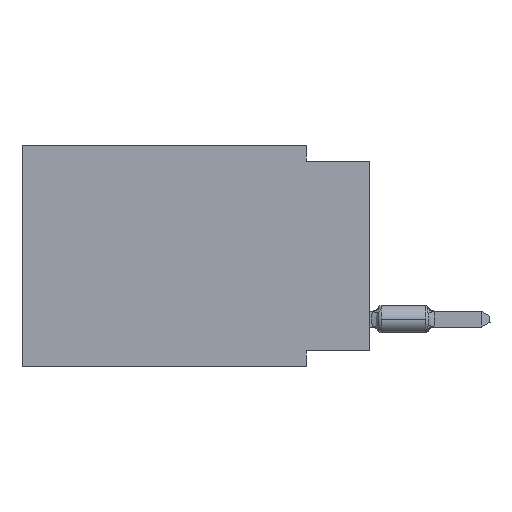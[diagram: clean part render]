
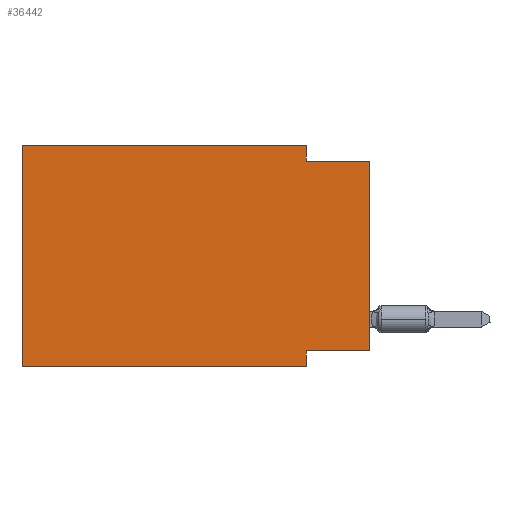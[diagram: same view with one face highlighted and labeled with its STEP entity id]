
A CAD part, left-side view. The second image highlights one B-rep face of the part: STEP entity #36442.
In plain terms, the highlighted planar face has unit normal (-1, 0, 0).
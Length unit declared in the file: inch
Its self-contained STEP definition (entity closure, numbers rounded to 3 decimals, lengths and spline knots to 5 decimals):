
#2089 = CARTESIAN_POINT ( 'NONE',  ( 0., 0.55, 0. ) ) ;
#2874 = EDGE_LOOP ( 'NONE', ( #9524, #22324, #49811, #8114, #31457, #65400, #49393, #23720 ) ) ;
#2951 = VECTOR ( 'NONE', #19163, 39.37008 ) ;
#5029 = EDGE_CURVE ( 'NONE', #24709, #63489, #42333, .T. ) ;
#6520 = CARTESIAN_POINT ( 'NONE',  ( 0., 0., -0.325 ) ) ;
#7232 = DIRECTION ( 'NONE',  ( 1., 0., 0. ) ) ;
#8114 = ORIENTED_EDGE ( 'NONE', *, *, #5029, .F. ) ;
#9524 = ORIENTED_EDGE ( 'NONE', *, *, #23085, .T. ) ;
#12585 = CARTESIAN_POINT ( 'NONE',  ( 0., 0.55, -0.35 ) ) ;
#13055 = DIRECTION ( 'NONE',  ( 0., 1., 0. ) ) ;
#14767 = LINE ( 'NONE', #37087, #65065 ) ;
#14959 = VECTOR ( 'NONE', #50602, 39.37008 ) ;
#18483 = EDGE_CURVE ( 'NONE', #66449, #24709, #29270, .T. ) ;
#18744 = VERTEX_POINT ( 'NONE', #65850 ) ;
#19163 = DIRECTION ( 'NONE',  ( 0., -1., 0. ) ) ;
#19245 = CARTESIAN_POINT ( 'NONE',  ( 0., 0.55, -0.35 ) ) ;
#20699 = CARTESIAN_POINT ( 'NONE',  ( 0., 0.1, -0.35 ) ) ;
#22324 = ORIENTED_EDGE ( 'NONE', *, *, #37115, .F. ) ;
#23085 = EDGE_CURVE ( 'NONE', #18744, #41054, #41085, .T. ) ;
#23563 = DIRECTION ( 'NONE',  ( 0., 0., 1. ) ) ;
#23720 = ORIENTED_EDGE ( 'NONE', *, *, #67613, .F. ) ;
#24709 = VERTEX_POINT ( 'NONE', #68118 ) ;
#26183 = LINE ( 'NONE', #20699, #42699 ) ;
#28802 = LINE ( 'NONE', #6520, #55781 ) ;
#29270 = LINE ( 'NONE', #47551, #40242 ) ;
#29521 = DIRECTION ( 'NONE',  ( 0., 0., -1. ) ) ;
#31457 = ORIENTED_EDGE ( 'NONE', *, *, #18483, .F. ) ;
#32283 = AXIS2_PLACEMENT_3D ( 'NONE', #41573, #7232, #29521 ) ;
#35723 = EDGE_CURVE ( 'NONE', #66449, #66657, #62725, .T. ) ;
#36092 = DIRECTION ( 'NONE',  ( 0., -1., 0. ) ) ;
#36442 = ADVANCED_FACE ( 'NONE', ( #47077 ), #42318, .F. ) ;
#36537 = VERTEX_POINT ( 'NONE', #66095 ) ;
#37087 = CARTESIAN_POINT ( 'NONE',  ( 0., 0., -0.025 ) ) ;
#37115 = EDGE_CURVE ( 'NONE', #46464, #41054, #14767, .T. ) ;
#37152 = VECTOR ( 'NONE', #23563, 39.37008 ) ;
#40242 = VECTOR ( 'NONE', #47922, 39.37008 ) ;
#41054 = VERTEX_POINT ( 'NONE', #60706 ) ;
#41085 = LINE ( 'NONE', #46952, #37152 ) ;
#41573 = CARTESIAN_POINT ( 'NONE',  ( 0., 0.55, 0. ) ) ;
#42318 = PLANE ( 'NONE',  #32283 ) ;
#42333 = LINE ( 'NONE', #2089, #64737 ) ;
#42699 = VECTOR ( 'NONE', #60564, 39.37008 ) ;
#45073 = CARTESIAN_POINT ( 'NONE',  ( 0., 0.1, 0. ) ) ;
#45833 = CARTESIAN_POINT ( 'NONE',  ( 0., 0.1, 0. ) ) ;
#46464 = VERTEX_POINT ( 'NONE', #51470 ) ;
#46952 = CARTESIAN_POINT ( 'NONE',  ( 0., 0., 0. ) ) ;
#47077 = FACE_OUTER_BOUND ( 'NONE', #2874, .T. ) ;
#47551 = CARTESIAN_POINT ( 'NONE',  ( 0., 0.55, 0. ) ) ;
#47922 = DIRECTION ( 'NONE',  ( 0., 0., 1. ) ) ;
#48459 = DIRECTION ( 'NONE',  ( 0., -1., 0. ) ) ;
#49393 = ORIENTED_EDGE ( 'NONE', *, *, #56763, .F. ) ;
#49811 = ORIENTED_EDGE ( 'NONE', *, *, #68405, .F. ) ;
#50602 = DIRECTION ( 'NONE',  ( 0., 0., -1. ) ) ;
#51470 = CARTESIAN_POINT ( 'NONE',  ( 0., 0.1, -0.025 ) ) ;
#55781 = VECTOR ( 'NONE', #13055, 39.37008 ) ;
#56763 = EDGE_CURVE ( 'NONE', #36537, #66657, #26183, .T. ) ;
#60564 = DIRECTION ( 'NONE',  ( 0., 0., -1. ) ) ;
#60706 = CARTESIAN_POINT ( 'NONE',  ( 0., 0., -0.025 ) ) ;
#61304 = CARTESIAN_POINT ( 'NONE',  ( 0., 0.1, -0.35 ) ) ;
#62725 = LINE ( 'NONE', #12585, #2951 ) ;
#63010 = LINE ( 'NONE', #45833, #14959 ) ;
#63489 = VERTEX_POINT ( 'NONE', #45073 ) ;
#64737 = VECTOR ( 'NONE', #36092, 39.37008 ) ;
#65065 = VECTOR ( 'NONE', #48459, 39.37008 ) ;
#65400 = ORIENTED_EDGE ( 'NONE', *, *, #35723, .T. ) ;
#65850 = CARTESIAN_POINT ( 'NONE',  ( 0., 0., -0.325 ) ) ;
#66095 = CARTESIAN_POINT ( 'NONE',  ( 0., 0.1, -0.325 ) ) ;
#66449 = VERTEX_POINT ( 'NONE', #19245 ) ;
#66657 = VERTEX_POINT ( 'NONE', #61304 ) ;
#67613 = EDGE_CURVE ( 'NONE', #18744, #36537, #28802, .T. ) ;
#68118 = CARTESIAN_POINT ( 'NONE',  ( 0., 0.55, 0. ) ) ;
#68405 = EDGE_CURVE ( 'NONE', #63489, #46464, #63010, .T. ) ;
